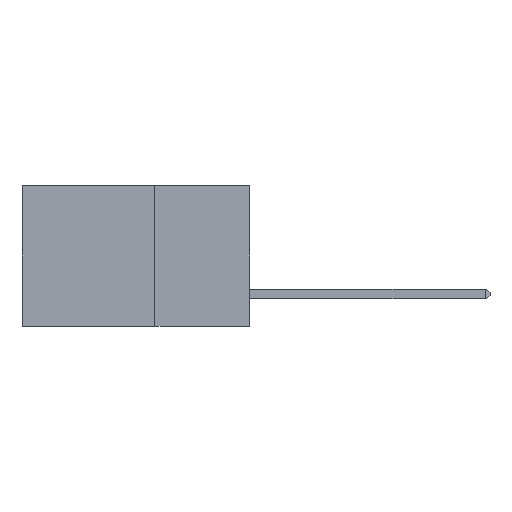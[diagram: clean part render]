
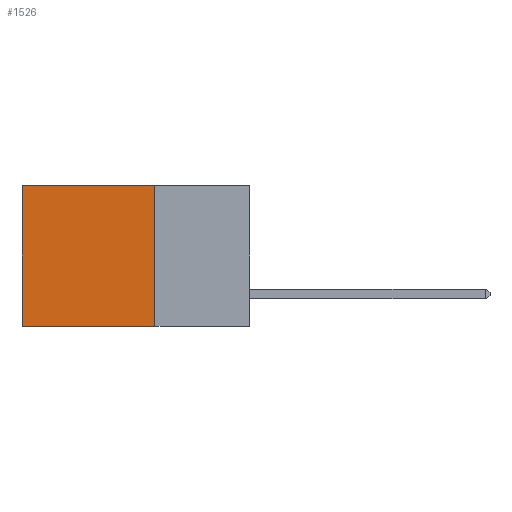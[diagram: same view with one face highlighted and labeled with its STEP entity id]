
A CAD part, left-side view. The second image highlights one B-rep face of the part: STEP entity #1526.
In plain terms, the highlighted planar face has unit normal (-1, 0, 0).
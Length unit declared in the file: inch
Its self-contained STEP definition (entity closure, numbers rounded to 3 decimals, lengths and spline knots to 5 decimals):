
#125 = ORIENTED_EDGE ( 'NONE', *, *, #3455, .F. ) ;
#836 = EDGE_CURVE ( 'NONE', #10283, #3420, #7276, .T. ) ;
#838 = PLANE ( 'NONE',  #11826 ) ;
#925 = CARTESIAN_POINT ( 'NONE',  ( 0.2875, 0.25, 0. ) ) ;
#1336 = CARTESIAN_POINT ( 'NONE',  ( 0.2875, 0.25, 0. ) ) ;
#1423 = VECTOR ( 'NONE', #12064, 39.37008 ) ;
#1526 = ADVANCED_FACE ( 'NONE', ( #10440 ), #838, .F. ) ;
#1653 = ORIENTED_EDGE ( 'NONE', *, *, #1914, .T. ) ;
#1746 = LINE ( 'NONE', #5639, #7362 ) ;
#1798 = DIRECTION ( 'NONE',  ( 0., 1., 0. ) ) ;
#1914 = EDGE_CURVE ( 'NONE', #12859, #10283, #3501, .T. ) ;
#2991 = EDGE_CURVE ( 'NONE', #12859, #10270, #4287, .T. ) ;
#3133 = CARTESIAN_POINT ( 'NONE',  ( 0.2875, 0.25, 0. ) ) ;
#3420 = VERTEX_POINT ( 'NONE', #9687 ) ;
#3455 = EDGE_CURVE ( 'NONE', #10270, #3420, #1746, .T. ) ;
#3501 = LINE ( 'NONE', #1336, #8690 ) ;
#4287 = LINE ( 'NONE', #11308, #1423 ) ;
#4520 = VECTOR ( 'NONE', #10039, 39.37008 ) ;
#4899 = DIRECTION ( 'NONE',  ( 0., 0., -1. ) ) ;
#5198 = CARTESIAN_POINT ( 'NONE',  ( 0.2875, 0.6, 0. ) ) ;
#5538 = DIRECTION ( 'NONE',  ( 0., 1., 0. ) ) ;
#5590 = ORIENTED_EDGE ( 'NONE', *, *, #836, .T. ) ;
#5639 = CARTESIAN_POINT ( 'NONE',  ( 0.2875, 0.25, -0.37 ) ) ;
#7276 = LINE ( 'NONE', #5198, #4520 ) ;
#7362 = VECTOR ( 'NONE', #5538, 39.37008 ) ;
#7929 = CARTESIAN_POINT ( 'NONE',  ( 0.2875, 0.25, -0.37 ) ) ;
#8690 = VECTOR ( 'NONE', #1798, 39.37008 ) ;
#9599 = ORIENTED_EDGE ( 'NONE', *, *, #2991, .F. ) ;
#9687 = CARTESIAN_POINT ( 'NONE',  ( 0.2875, 0.6, -0.37 ) ) ;
#10034 = DIRECTION ( 'NONE',  ( 1., 0., 0. ) ) ;
#10039 = DIRECTION ( 'NONE',  ( 0., 0., -1. ) ) ;
#10270 = VERTEX_POINT ( 'NONE', #7929 ) ;
#10283 = VERTEX_POINT ( 'NONE', #12961 ) ;
#10358 = EDGE_LOOP ( 'NONE', ( #5590, #125, #9599, #1653 ) ) ;
#10440 = FACE_OUTER_BOUND ( 'NONE', #10358, .T. ) ;
#11308 = CARTESIAN_POINT ( 'NONE',  ( 0.2875, 0.25, 0. ) ) ;
#11826 = AXIS2_PLACEMENT_3D ( 'NONE', #3133, #10034, #4899 ) ;
#12064 = DIRECTION ( 'NONE',  ( 0., 0., -1. ) ) ;
#12859 = VERTEX_POINT ( 'NONE', #925 ) ;
#12961 = CARTESIAN_POINT ( 'NONE',  ( 0.2875, 0.6, 0. ) ) ;
